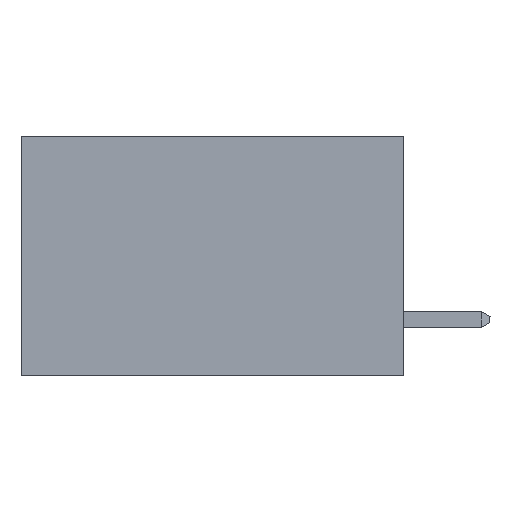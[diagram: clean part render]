
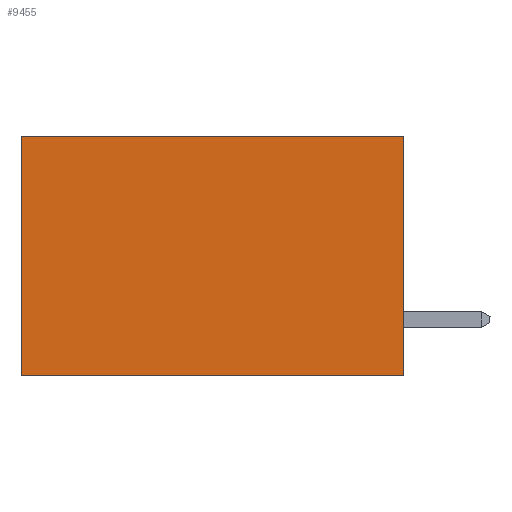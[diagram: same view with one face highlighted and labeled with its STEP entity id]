
A CAD part, left-side view. The second image highlights one B-rep face of the part: STEP entity #9455.
In plain terms, the highlighted planar face has unit normal (-1, 0, 0).
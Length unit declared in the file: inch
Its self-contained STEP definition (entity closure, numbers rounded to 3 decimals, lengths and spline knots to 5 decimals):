
#15 = ORIENTED_EDGE ( 'NONE', *, *, #6532, .T. ) ;
#262 = EDGE_CURVE ( 'NONE', #6624, #9040, #11863, .T. ) ;
#421 = EDGE_LOOP ( 'NONE', ( #15, #12824, #12288, #9897 ) ) ;
#670 = VERTEX_POINT ( 'NONE', #6951 ) ;
#721 = CARTESIAN_POINT ( 'NONE',  ( 0.2875, 0., -0.375 ) ) ;
#748 = DIRECTION ( 'NONE',  ( 0., 1., 0. ) ) ;
#853 = CARTESIAN_POINT ( 'NONE',  ( 0.2875, 0.6, -0.375 ) ) ;
#957 = CARTESIAN_POINT ( 'NONE',  ( 0.2875, 0.6, 0. ) ) ;
#1783 = CARTESIAN_POINT ( 'NONE',  ( 0.2875, 0., -0.375 ) ) ;
#1815 = DIRECTION ( 'NONE',  ( 0., 0., -1. ) ) ;
#2286 = EDGE_CURVE ( 'NONE', #670, #5673, #3688, .T. ) ;
#2362 = VECTOR ( 'NONE', #748, 39.37008 ) ;
#2452 = VECTOR ( 'NONE', #5761, 39.37008 ) ;
#2924 = DIRECTION ( 'NONE',  ( 0., 1., 0. ) ) ;
#3688 = LINE ( 'NONE', #9681, #2362 ) ;
#4755 = AXIS2_PLACEMENT_3D ( 'NONE', #721, #10625, #1815 ) ;
#4916 = LINE ( 'NONE', #1783, #2452 ) ;
#5602 = PLANE ( 'NONE',  #4755 ) ;
#5673 = VERTEX_POINT ( 'NONE', #957 ) ;
#5761 = DIRECTION ( 'NONE',  ( 0., 0., -1. ) ) ;
#6532 = EDGE_CURVE ( 'NONE', #5673, #9040, #9468, .T. ) ;
#6624 = VERTEX_POINT ( 'NONE', #11022 ) ;
#6708 = CARTESIAN_POINT ( 'NONE',  ( 0.2875, 0.6, -0.375 ) ) ;
#6896 = CARTESIAN_POINT ( 'NONE',  ( 0.2875, 0., -0.375 ) ) ;
#6951 = CARTESIAN_POINT ( 'NONE',  ( 0.2875, 0., 0. ) ) ;
#9040 = VERTEX_POINT ( 'NONE', #853 ) ;
#9230 = VECTOR ( 'NONE', #10439, 39.37008 ) ;
#9455 = ADVANCED_FACE ( 'NONE', ( #10563 ), #5602, .F. ) ;
#9468 = LINE ( 'NONE', #6708, #9230 ) ;
#9681 = CARTESIAN_POINT ( 'NONE',  ( 0.2875, 0., 0. ) ) ;
#9897 = ORIENTED_EDGE ( 'NONE', *, *, #2286, .T. ) ;
#10410 = EDGE_CURVE ( 'NONE', #670, #6624, #4916, .T. ) ;
#10439 = DIRECTION ( 'NONE',  ( 0., 0., -1. ) ) ;
#10563 = FACE_OUTER_BOUND ( 'NONE', #421, .T. ) ;
#10625 = DIRECTION ( 'NONE',  ( 1., 0., 0. ) ) ;
#11022 = CARTESIAN_POINT ( 'NONE',  ( 0.2875, 0., -0.375 ) ) ;
#11380 = VECTOR ( 'NONE', #2924, 39.37008 ) ;
#11863 = LINE ( 'NONE', #6896, #11380 ) ;
#12288 = ORIENTED_EDGE ( 'NONE', *, *, #10410, .F. ) ;
#12824 = ORIENTED_EDGE ( 'NONE', *, *, #262, .F. ) ;
